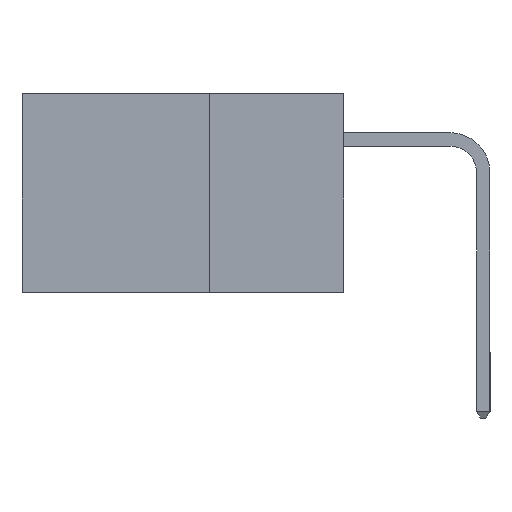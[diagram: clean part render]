
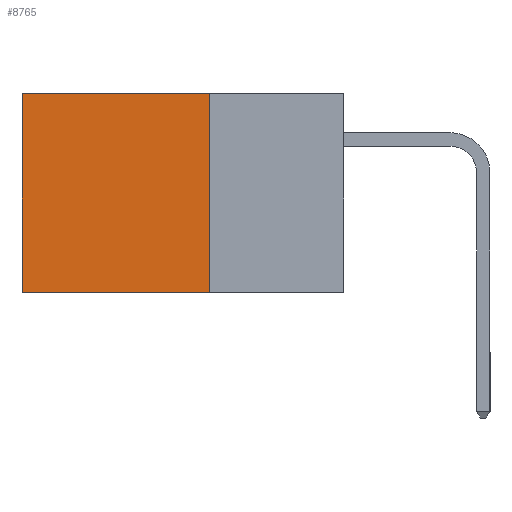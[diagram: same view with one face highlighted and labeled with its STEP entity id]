
A CAD part, left-side view. The second image highlights one B-rep face of the part: STEP entity #8765.
In plain terms, the highlighted planar face has unit normal (-1, 0, 0).
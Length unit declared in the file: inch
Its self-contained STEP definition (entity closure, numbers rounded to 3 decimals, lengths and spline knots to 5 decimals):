
#2149 = EDGE_CURVE ( 'NONE', #15668, #5869, #16433, .T. ) ;
#2399 = CARTESIAN_POINT ( 'NONE',  ( 0.298, 0.6, -0.37 ) ) ;
#2767 = AXIS2_PLACEMENT_3D ( 'NONE', #5863, #13021, #14515 ) ;
#3682 = FACE_OUTER_BOUND ( 'NONE', #3851, .T. ) ;
#3778 = VECTOR ( 'NONE', #18409, 39.37008 ) ;
#3851 = EDGE_LOOP ( 'NONE', ( #13755, #10211, #8122, #16123 ) ) ;
#3944 = EDGE_CURVE ( 'NONE', #13742, #8235, #14065, .T. ) ;
#5072 = LINE ( 'NONE', #16430, #16324 ) ;
#5115 = EDGE_CURVE ( 'NONE', #8235, #5869, #5072, .T. ) ;
#5120 = CARTESIAN_POINT ( 'NONE',  ( 0.298, 0.25, -0.37 ) ) ;
#5863 = CARTESIAN_POINT ( 'NONE',  ( 0.298, 0.25, 0. ) ) ;
#5869 = VERTEX_POINT ( 'NONE', #2399 ) ;
#8082 = PLANE ( 'NONE',  #2767 ) ;
#8122 = ORIENTED_EDGE ( 'NONE', *, *, #16168, .F. ) ;
#8235 = VERTEX_POINT ( 'NONE', #16912 ) ;
#8765 = ADVANCED_FACE ( 'NONE', ( #3682 ), #8082, .F. ) ;
#8829 = VECTOR ( 'NONE', #9510, 39.37008 ) ;
#9212 = DIRECTION ( 'NONE',  ( 0., 0., -1. ) ) ;
#9510 = DIRECTION ( 'NONE',  ( 0., 1., 0. ) ) ;
#10211 = ORIENTED_EDGE ( 'NONE', *, *, #2149, .F. ) ;
#11009 = CARTESIAN_POINT ( 'NONE',  ( 0.298, 0.25, 0. ) ) ;
#13021 = DIRECTION ( 'NONE',  ( 1., 0., 0. ) ) ;
#13687 = DIRECTION ( 'NONE',  ( 0., 0., -1. ) ) ;
#13742 = VERTEX_POINT ( 'NONE', #13881 ) ;
#13755 = ORIENTED_EDGE ( 'NONE', *, *, #5115, .T. ) ;
#13881 = CARTESIAN_POINT ( 'NONE',  ( 0.298, 0.25, 0. ) ) ;
#14065 = LINE ( 'NONE', #15667, #3778 ) ;
#14076 = CARTESIAN_POINT ( 'NONE',  ( 0.298, 0.25, -0.37 ) ) ;
#14515 = DIRECTION ( 'NONE',  ( 0., 0., -1. ) ) ;
#15667 = CARTESIAN_POINT ( 'NONE',  ( 0.298, 0.25, 0. ) ) ;
#15668 = VERTEX_POINT ( 'NONE', #5120 ) ;
#15786 = LINE ( 'NONE', #11009, #16674 ) ;
#16123 = ORIENTED_EDGE ( 'NONE', *, *, #3944, .T. ) ;
#16168 = EDGE_CURVE ( 'NONE', #13742, #15668, #15786, .T. ) ;
#16324 = VECTOR ( 'NONE', #9212, 39.37008 ) ;
#16430 = CARTESIAN_POINT ( 'NONE',  ( 0.298, 0.6, 0. ) ) ;
#16433 = LINE ( 'NONE', #14076, #8829 ) ;
#16674 = VECTOR ( 'NONE', #13687, 39.37008 ) ;
#16912 = CARTESIAN_POINT ( 'NONE',  ( 0.298, 0.6, 0. ) ) ;
#18409 = DIRECTION ( 'NONE',  ( 0., 1., 0. ) ) ;
